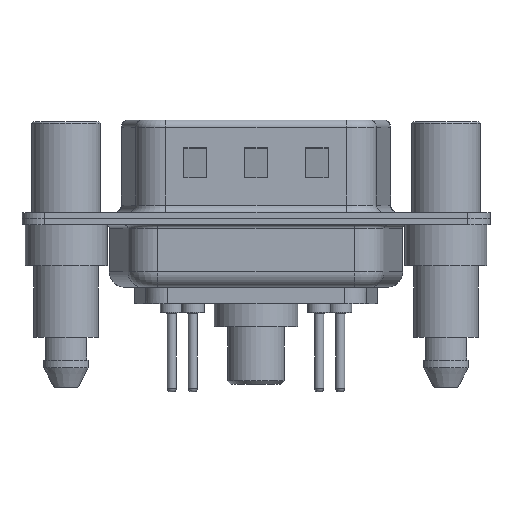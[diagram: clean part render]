
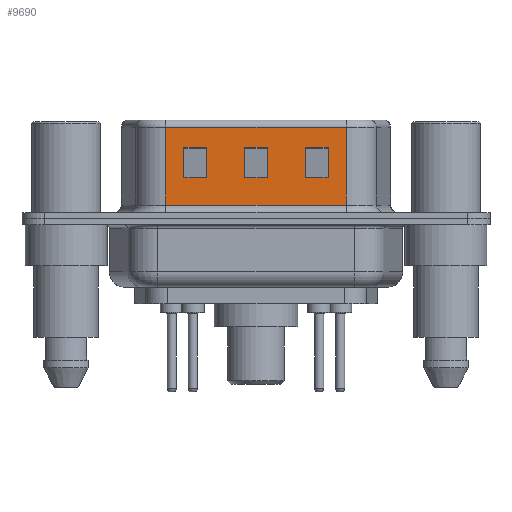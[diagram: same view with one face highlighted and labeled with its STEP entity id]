
A CAD part, front view. The second image highlights one B-rep face of the part: STEP entity #9690.
In plain terms, the highlighted planar face has unit normal (0, -1, 0).
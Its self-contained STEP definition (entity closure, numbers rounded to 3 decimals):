
#102 = DIRECTION ( 'NONE',  ( -1., 0., 0. ) ) ;
#113 = CARTESIAN_POINT ( 'NONE',  ( 6.55, -4.58, 6.02 ) ) ;
#117 = DIRECTION ( 'NONE',  ( -1., 0., 0. ) ) ;
#204 = ORIENTED_EDGE ( 'NONE', *, *, #5505, .T. ) ;
#525 = ORIENTED_EDGE ( 'NONE', *, *, #15736, .T. ) ;
#530 = EDGE_CURVE ( 'NONE', #9968, #4687, #801, .T. ) ;
#761 = CARTESIAN_POINT ( 'NONE',  ( 15.75, -4.58, 4.705 ) ) ;
#764 = VECTOR ( 'NONE', #15390, 1000. ) ;
#801 = LINE ( 'NONE', #9716, #11154 ) ;
#840 = CARTESIAN_POINT ( 'NONE',  ( 11.75, -4.58, 6.52 ) ) ;
#859 = EDGE_CURVE ( 'NONE', #9769, #4700, #9017, .T. ) ;
#928 = CARTESIAN_POINT ( 'NONE',  ( 22.45, -4.58, 2.705 ) ) ;
#1286 = CARTESIAN_POINT ( 'NONE',  ( 13.25, -4.58, 4.705 ) ) ;
#1343 = CARTESIAN_POINT ( 'NONE',  ( 14.45, -4.58, 4.705 ) ) ;
#1387 = CARTESIAN_POINT ( 'NONE',  ( 6.55, -4.58, 0.9 ) ) ;
#1398 = DIRECTION ( 'NONE',  ( 1., 0., 0. ) ) ;
#1580 = VECTOR ( 'NONE', #117, 1000. ) ;
#1601 = VECTOR ( 'NONE', #12073, 1000. ) ;
#1682 = ORIENTED_EDGE ( 'NONE', *, *, #530, .T. ) ;
#2248 = VECTOR ( 'NONE', #11799, 1000. ) ;
#2291 = DIRECTION ( 'NONE',  ( -1., 0., 0. ) ) ;
#2390 = CARTESIAN_POINT ( 'NONE',  ( 17.25, -4.58, 6.52 ) ) ;
#2470 = PLANE ( 'NONE',  #13916 ) ;
#2471 = CARTESIAN_POINT ( 'NONE',  ( 9.25, -4.58, 2.705 ) ) ;
#2648 = CARTESIAN_POINT ( 'NONE',  ( 11.75, -4.58, 4.705 ) ) ;
#2701 = LINE ( 'NONE', #928, #15837 ) ;
#2876 = ORIENTED_EDGE ( 'NONE', *, *, #12945, .T. ) ;
#3113 = CARTESIAN_POINT ( 'NONE',  ( 18.45, -4.58, 6.02 ) ) ;
#3174 = FACE_BOUND ( 'NONE', #3208, .T. ) ;
#3208 = EDGE_LOOP ( 'NONE', ( #17294, #4676, #525, #2876 ) ) ;
#3314 = LINE ( 'NONE', #1343, #6447 ) ;
#3491 = EDGE_LOOP ( 'NONE', ( #6219, #4616, #1682, #6572 ) ) ;
#3526 = LINE ( 'NONE', #14042, #14337 ) ;
#3599 = VECTOR ( 'NONE', #102, 1000. ) ;
#3690 = EDGE_CURVE ( 'NONE', #7471, #7432, #3526, .T. ) ;
#4027 = EDGE_CURVE ( 'NONE', #7432, #7286, #3314, .T. ) ;
#4057 = VERTEX_POINT ( 'NONE', #4870 ) ;
#4199 = EDGE_CURVE ( 'NONE', #12685, #13960, #11527, .T. ) ;
#4383 = LINE ( 'NONE', #11276, #17604 ) ;
#4397 = CARTESIAN_POINT ( 'NONE',  ( 9.25, -4.58, 4.705 ) ) ;
#4463 = EDGE_CURVE ( 'NONE', #9375, #9769, #5398, .T. ) ;
#4616 = ORIENTED_EDGE ( 'NONE', *, *, #13796, .T. ) ;
#4676 = ORIENTED_EDGE ( 'NONE', *, *, #859, .T. ) ;
#4687 = VERTEX_POINT ( 'NONE', #761 ) ;
#4700 = VERTEX_POINT ( 'NONE', #15548 ) ;
#4780 = VECTOR ( 'NONE', #6241, 1000. ) ;
#4866 = ORIENTED_EDGE ( 'NONE', *, *, #12489, .T. ) ;
#4870 = CARTESIAN_POINT ( 'NONE',  ( 17.25, -4.58, 2.705 ) ) ;
#5153 = LINE ( 'NONE', #7043, #15587 ) ;
#5310 = ORIENTED_EDGE ( 'NONE', *, *, #9107, .T. ) ;
#5398 = LINE ( 'NONE', #11138, #15414 ) ;
#5505 = EDGE_CURVE ( 'NONE', #7286, #6349, #15588, .T. ) ;
#5536 = LINE ( 'NONE', #11087, #15541 ) ;
#5983 = CARTESIAN_POINT ( 'NONE',  ( 9.25, -4.58, 6.52 ) ) ;
#6219 = ORIENTED_EDGE ( 'NONE', *, *, #14368, .T. ) ;
#6241 = DIRECTION ( 'NONE',  ( 0., 0., 1. ) ) ;
#6349 = VERTEX_POINT ( 'NONE', #2471 ) ;
#6447 = VECTOR ( 'NONE', #1398, 1000. ) ;
#6505 = DIRECTION ( 'NONE',  ( 0., 1., 0. ) ) ;
#6572 = ORIENTED_EDGE ( 'NONE', *, *, #11698, .T. ) ;
#7043 = CARTESIAN_POINT ( 'NONE',  ( 18.45, -4.58, 6.52 ) ) ;
#7286 = VERTEX_POINT ( 'NONE', #4397 ) ;
#7432 = VERTEX_POINT ( 'NONE', #16001 ) ;
#7471 = VERTEX_POINT ( 'NONE', #14386 ) ;
#7511 = EDGE_CURVE ( 'NONE', #14530, #12036, #5536, .T. ) ;
#8206 = EDGE_LOOP ( 'NONE', ( #204, #5310, #8602, #9291 ) ) ;
#8217 = FACE_BOUND ( 'NONE', #3491, .T. ) ;
#8602 = ORIENTED_EDGE ( 'NONE', *, *, #3690, .T. ) ;
#8813 = DIRECTION ( 'NONE',  ( 0., 0., -1. ) ) ;
#8914 = DIRECTION ( 'NONE',  ( 1., 0., 0. ) ) ;
#9017 = LINE ( 'NONE', #16085, #14997 ) ;
#9107 = EDGE_CURVE ( 'NONE', #6349, #7471, #14846, .T. ) ;
#9291 = ORIENTED_EDGE ( 'NONE', *, *, #4027, .T. ) ;
#9375 = VERTEX_POINT ( 'NONE', #2648 ) ;
#9500 = ORIENTED_EDGE ( 'NONE', *, *, #15170, .F. ) ;
#9690 = ADVANCED_FACE ( 'NONE', ( #17190, #8217, #3174, #13518 ), #2470, .F. ) ;
#9716 = CARTESIAN_POINT ( 'NONE',  ( 15.75, -4.58, 6.52 ) ) ;
#9769 = VERTEX_POINT ( 'NONE', #1286 ) ;
#9962 = DIRECTION ( 'NONE',  ( 1., 0., 0. ) ) ;
#9968 = VERTEX_POINT ( 'NONE', #16523 ) ;
#11054 = EDGE_LOOP ( 'NONE', ( #9500, #13530, #4866, #12086 ) ) ;
#11058 = CARTESIAN_POINT ( 'NONE',  ( 18.45, -4.58, 6.02 ) ) ;
#11087 = CARTESIAN_POINT ( 'NONE',  ( 18.45, -4.58, 0.9 ) ) ;
#11138 = CARTESIAN_POINT ( 'NONE',  ( 18.45, -4.58, 4.705 ) ) ;
#11154 = VECTOR ( 'NONE', #11207, 1000. ) ;
#11207 = DIRECTION ( 'NONE',  ( 0., 0., 1. ) ) ;
#11276 = CARTESIAN_POINT ( 'NONE',  ( 22.45, -4.58, 4.705 ) ) ;
#11527 = LINE ( 'NONE', #3113, #764 ) ;
#11698 = EDGE_CURVE ( 'NONE', #4687, #16694, #4383, .T. ) ;
#11799 = DIRECTION ( 'NONE',  ( 0., 0., -1. ) ) ;
#11938 = DIRECTION ( 'NONE',  ( 0., 0., 1. ) ) ;
#12036 = VERTEX_POINT ( 'NONE', #13262 ) ;
#12073 = DIRECTION ( 'NONE',  ( 0., 0., -1. ) ) ;
#12086 = ORIENTED_EDGE ( 'NONE', *, *, #7511, .T. ) ;
#12141 = CARTESIAN_POINT ( 'NONE',  ( 14.45, -4.58, 2.705 ) ) ;
#12174 = CARTESIAN_POINT ( 'NONE',  ( 18.45, -4.58, 2.705 ) ) ;
#12489 = EDGE_CURVE ( 'NONE', #13960, #14530, #14373, .T. ) ;
#12577 = LINE ( 'NONE', #2390, #2248 ) ;
#12685 = VERTEX_POINT ( 'NONE', #11058 ) ;
#12945 = EDGE_CURVE ( 'NONE', #16816, #9375, #15642, .T. ) ;
#13262 = CARTESIAN_POINT ( 'NONE',  ( 18.45, -4.58, 0.9 ) ) ;
#13518 = FACE_OUTER_BOUND ( 'NONE', #11054, .T. ) ;
#13526 = DIRECTION ( 'NONE',  ( 0., 0., -1. ) ) ;
#13530 = ORIENTED_EDGE ( 'NONE', *, *, #4199, .T. ) ;
#13796 = EDGE_CURVE ( 'NONE', #4057, #9968, #2701, .T. ) ;
#13916 = AXIS2_PLACEMENT_3D ( 'NONE', #14553, #6505, #16059 ) ;
#13948 = VECTOR ( 'NONE', #8813, 1000. ) ;
#13960 = VERTEX_POINT ( 'NONE', #113 ) ;
#14042 = CARTESIAN_POINT ( 'NONE',  ( 7.75, -4.58, 6.52 ) ) ;
#14337 = VECTOR ( 'NONE', #11938, 1000. ) ;
#14368 = EDGE_CURVE ( 'NONE', #16694, #4057, #12577, .T. ) ;
#14373 = LINE ( 'NONE', #15572, #13948 ) ;
#14386 = CARTESIAN_POINT ( 'NONE',  ( 7.75, -4.58, 2.705 ) ) ;
#14530 = VERTEX_POINT ( 'NONE', #1387 ) ;
#14553 = CARTESIAN_POINT ( 'NONE',  ( 18.45, -4.58, 6.52 ) ) ;
#14846 = LINE ( 'NONE', #12141, #3599 ) ;
#14997 = VECTOR ( 'NONE', #13526, 1000. ) ;
#15170 = EDGE_CURVE ( 'NONE', #12685, #12036, #5153, .T. ) ;
#15275 = DIRECTION ( 'NONE',  ( 0., 0., -1. ) ) ;
#15390 = DIRECTION ( 'NONE',  ( -1., 0., 0. ) ) ;
#15414 = VECTOR ( 'NONE', #8914, 1000. ) ;
#15541 = VECTOR ( 'NONE', #17567, 1000. ) ;
#15548 = CARTESIAN_POINT ( 'NONE',  ( 13.25, -4.58, 2.705 ) ) ;
#15572 = CARTESIAN_POINT ( 'NONE',  ( 6.55, -4.58, 6.52 ) ) ;
#15587 = VECTOR ( 'NONE', #15275, 1000. ) ;
#15588 = LINE ( 'NONE', #5983, #1601 ) ;
#15642 = LINE ( 'NONE', #840, #4780 ) ;
#15736 = EDGE_CURVE ( 'NONE', #4700, #16816, #16007, .T. ) ;
#15837 = VECTOR ( 'NONE', #2291, 1000. ) ;
#15888 = CARTESIAN_POINT ( 'NONE',  ( 17.25, -4.58, 4.705 ) ) ;
#16001 = CARTESIAN_POINT ( 'NONE',  ( 7.75, -4.58, 4.705 ) ) ;
#16007 = LINE ( 'NONE', #12174, #1580 ) ;
#16059 = DIRECTION ( 'NONE',  ( 0., 0., 1. ) ) ;
#16085 = CARTESIAN_POINT ( 'NONE',  ( 13.25, -4.58, 6.52 ) ) ;
#16523 = CARTESIAN_POINT ( 'NONE',  ( 15.75, -4.58, 2.705 ) ) ;
#16694 = VERTEX_POINT ( 'NONE', #15888 ) ;
#16816 = VERTEX_POINT ( 'NONE', #17452 ) ;
#17190 = FACE_BOUND ( 'NONE', #8206, .T. ) ;
#17294 = ORIENTED_EDGE ( 'NONE', *, *, #4463, .T. ) ;
#17452 = CARTESIAN_POINT ( 'NONE',  ( 11.75, -4.58, 2.705 ) ) ;
#17567 = DIRECTION ( 'NONE',  ( 1., 0., 0. ) ) ;
#17604 = VECTOR ( 'NONE', #9962, 1000. ) ;
